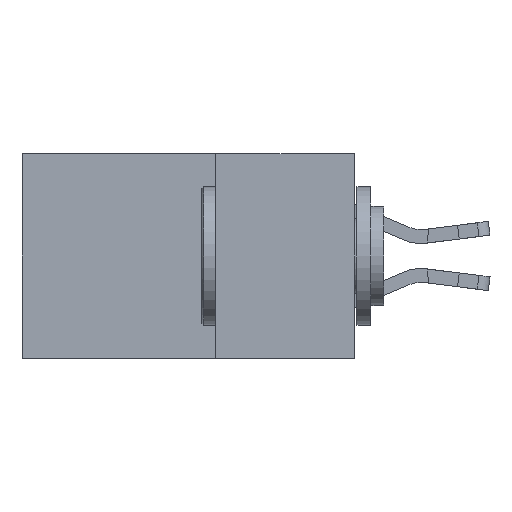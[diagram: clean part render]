
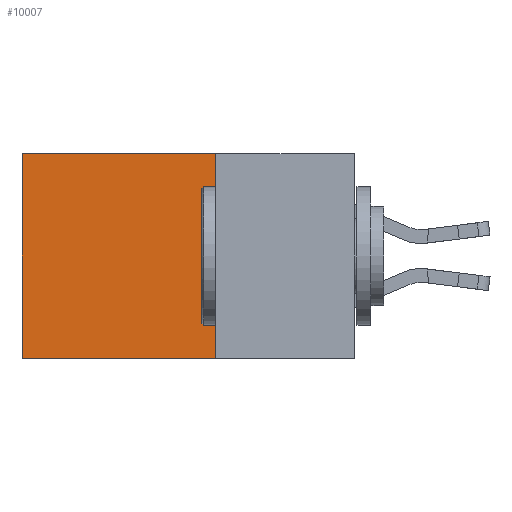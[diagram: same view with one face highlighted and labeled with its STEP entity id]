
A CAD part, left-side view. The second image highlights one B-rep face of the part: STEP entity #10007.
In plain terms, the highlighted planar face has unit normal (-1, 0, 0).
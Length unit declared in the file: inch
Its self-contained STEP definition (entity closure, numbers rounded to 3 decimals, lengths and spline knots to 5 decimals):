
#165 = ORIENTED_EDGE ( 'NONE', *, *, #9803, .T. ) ;
#197 = LINE ( 'NONE', #8566, #3422 ) ;
#1046 = CARTESIAN_POINT ( 'NONE',  ( 0.298, 0.6, 0. ) ) ;
#1743 = EDGE_CURVE ( 'NONE', #6414, #17318, #1917, .T. ) ;
#1917 = LINE ( 'NONE', #3084, #16150 ) ;
#2049 = DIRECTION ( 'NONE',  ( 0., 0., -1. ) ) ;
#3084 = CARTESIAN_POINT ( 'NONE',  ( 0.298, 0.25, 0. ) ) ;
#3422 = VECTOR ( 'NONE', #7766, 39.37008 ) ;
#4814 = EDGE_CURVE ( 'NONE', #6414, #11486, #197, .T. ) ;
#5430 = DIRECTION ( 'NONE',  ( 0., 0., -1. ) ) ;
#5504 = ORIENTED_EDGE ( 'NONE', *, *, #14407, .F. ) ;
#5507 = CARTESIAN_POINT ( 'NONE',  ( 0.298, 0.6, -0.37 ) ) ;
#5814 = AXIS2_PLACEMENT_3D ( 'NONE', #8918, #8801, #2049 ) ;
#6414 = VERTEX_POINT ( 'NONE', #15778 ) ;
#6772 = CARTESIAN_POINT ( 'NONE',  ( 0.298, 0.6, 0. ) ) ;
#7602 = PLANE ( 'NONE',  #5814 ) ;
#7766 = DIRECTION ( 'NONE',  ( 0., 1., 0. ) ) ;
#7891 = LINE ( 'NONE', #6772, #15138 ) ;
#7960 = ORIENTED_EDGE ( 'NONE', *, *, #1743, .F. ) ;
#8081 = CARTESIAN_POINT ( 'NONE',  ( 0.298, 0.25, -0.37 ) ) ;
#8566 = CARTESIAN_POINT ( 'NONE',  ( 0.298, 0.25, 0. ) ) ;
#8801 = DIRECTION ( 'NONE',  ( 1., 0., 0. ) ) ;
#8918 = CARTESIAN_POINT ( 'NONE',  ( 0.298, 0.25, 0. ) ) ;
#9737 = DIRECTION ( 'NONE',  ( 0., 1., 0. ) ) ;
#9803 = EDGE_CURVE ( 'NONE', #11486, #15294, #7891, .T. ) ;
#9998 = DIRECTION ( 'NONE',  ( 0., 0., -1. ) ) ;
#10007 = ADVANCED_FACE ( 'NONE', ( #10043 ), #7602, .F. ) ;
#10043 = FACE_OUTER_BOUND ( 'NONE', #11198, .T. ) ;
#11072 = CARTESIAN_POINT ( 'NONE',  ( 0.298, 0.25, -0.37 ) ) ;
#11198 = EDGE_LOOP ( 'NONE', ( #165, #5504, #7960, #15234 ) ) ;
#11486 = VERTEX_POINT ( 'NONE', #1046 ) ;
#14407 = EDGE_CURVE ( 'NONE', #17318, #15294, #17631, .T. ) ;
#15138 = VECTOR ( 'NONE', #5430, 39.37008 ) ;
#15234 = ORIENTED_EDGE ( 'NONE', *, *, #4814, .T. ) ;
#15294 = VERTEX_POINT ( 'NONE', #5507 ) ;
#15778 = CARTESIAN_POINT ( 'NONE',  ( 0.298, 0.25, 0. ) ) ;
#16150 = VECTOR ( 'NONE', #9998, 39.37008 ) ;
#16313 = VECTOR ( 'NONE', #9737, 39.37008 ) ;
#17318 = VERTEX_POINT ( 'NONE', #8081 ) ;
#17631 = LINE ( 'NONE', #11072, #16313 ) ;
